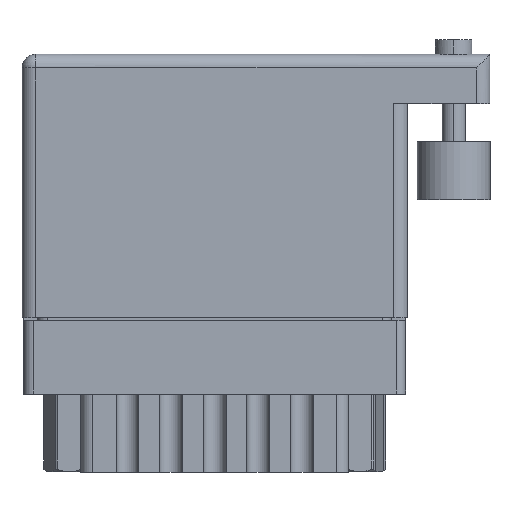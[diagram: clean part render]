
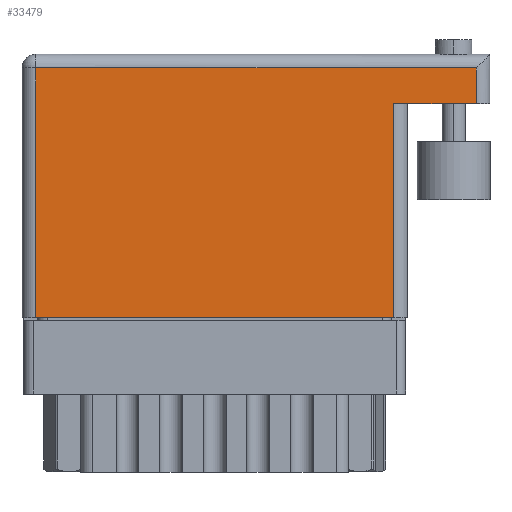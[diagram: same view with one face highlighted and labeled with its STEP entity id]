
A CAD part, front view. The second image highlights one B-rep face of the part: STEP entity #33479.
In plain terms, the highlighted face is planar.
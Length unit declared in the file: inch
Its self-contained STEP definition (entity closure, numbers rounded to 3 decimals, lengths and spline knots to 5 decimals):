
#558 = ORIENTED_EDGE ( 'NONE', *, *, #15516, .T. ) ;
#745 = CARTESIAN_POINT ( 'NONE',  ( 0.047, 0., 0. ) ) ;
#746 = VECTOR ( 'NONE', #2773, 39.37008 ) ;
#1311 = CARTESIAN_POINT ( 'NONE',  ( 1.562, 0.736, 0. ) ) ;
#1581 = FACE_OUTER_BOUND ( 'NONE', #8295, .T. ) ;
#2638 = VECTOR ( 'NONE', #4875, 39.37008 ) ;
#2724 = ORIENTED_EDGE ( 'NONE', *, *, #6875, .T. ) ;
#2773 = DIRECTION ( 'NONE',  ( -1., 0., 0. ) ) ;
#3708 = VERTEX_POINT ( 'NONE', #17145 ) ;
#3915 = LINE ( 'NONE', #11828, #11677 ) ;
#4875 = DIRECTION ( 'NONE',  ( 1., 0., 0. ) ) ;
#6190 = DIRECTION ( 'NONE',  ( 0., -1., 0. ) ) ;
#6875 = EDGE_CURVE ( 'NONE', #28937, #33581, #33011, .T. ) ;
#8295 = EDGE_LOOP ( 'NONE', ( #2724, #34405, #11783, #15850, #558, #21733 ) ) ;
#8305 = CARTESIAN_POINT ( 'NONE',  ( 1.609, 0.736, 0. ) ) ;
#9118 = CARTESIAN_POINT ( 'NONE',  ( 0., 0.859, 0. ) ) ;
#9911 = CARTESIAN_POINT ( 'NONE',  ( 0., 0.906, 0. ) ) ;
#11050 = LINE ( 'NONE', #9118, #26688 ) ;
#11677 = VECTOR ( 'NONE', #17539, 39.37008 ) ;
#11783 = ORIENTED_EDGE ( 'NONE', *, *, #16370, .F. ) ;
#11828 = CARTESIAN_POINT ( 'NONE',  ( 1.562, 0.906, 0. ) ) ;
#12876 = VERTEX_POINT ( 'NONE', #16532 ) ;
#14589 = LINE ( 'NONE', #8305, #746 ) ;
#15516 = EDGE_CURVE ( 'NONE', #3708, #27680, #11050, .T. ) ;
#15619 = DIRECTION ( 'NONE',  ( 0., 0., -1. ) ) ;
#15850 = ORIENTED_EDGE ( 'NONE', *, *, #25641, .T. ) ;
#15923 = AXIS2_PLACEMENT_3D ( 'NONE', #9911, #15619, #21220 ) ;
#16338 = LINE ( 'NONE', #27416, #28926 ) ;
#16370 = EDGE_CURVE ( 'NONE', #19627, #12876, #14589, .T. ) ;
#16532 = CARTESIAN_POINT ( 'NONE',  ( 1.278, 0.736, 0. ) ) ;
#17021 = PLANE ( 'NONE',  #15923 ) ;
#17145 = CARTESIAN_POINT ( 'NONE',  ( 1.562, 0.859, 0. ) ) ;
#17539 = DIRECTION ( 'NONE',  ( 0., 1., 0. ) ) ;
#18424 = CARTESIAN_POINT ( 'NONE',  ( 1.278, 0., 0. ) ) ;
#18737 = CARTESIAN_POINT ( 'NONE',  ( 0.047, 0., 0. ) ) ;
#19627 = VERTEX_POINT ( 'NONE', #1311 ) ;
#21220 = DIRECTION ( 'NONE',  ( -1., 0., 0. ) ) ;
#21733 = ORIENTED_EDGE ( 'NONE', *, *, #23519, .T. ) ;
#23519 = EDGE_CURVE ( 'NONE', #27680, #28937, #23958, .T. ) ;
#23958 = LINE ( 'NONE', #745, #25241 ) ;
#24532 = CARTESIAN_POINT ( 'NONE',  ( 0.047, 0.859, 0. ) ) ;
#25241 = VECTOR ( 'NONE', #6190, 39.37008 ) ;
#25641 = EDGE_CURVE ( 'NONE', #19627, #3708, #3915, .T. ) ;
#26688 = VECTOR ( 'NONE', #28174, 39.37008 ) ;
#27416 = CARTESIAN_POINT ( 'NONE',  ( 1.278, 0.736, 0. ) ) ;
#27680 = VERTEX_POINT ( 'NONE', #24532 ) ;
#27748 = EDGE_CURVE ( 'NONE', #33581, #12876, #16338, .T. ) ;
#28174 = DIRECTION ( 'NONE',  ( -1., 0., 0. ) ) ;
#28926 = VECTOR ( 'NONE', #30322, 39.37008 ) ;
#28937 = VERTEX_POINT ( 'NONE', #18737 ) ;
#30322 = DIRECTION ( 'NONE',  ( 0., 1., 0. ) ) ;
#33011 = LINE ( 'NONE', #33124, #2638 ) ;
#33124 = CARTESIAN_POINT ( 'NONE',  ( 0., 0., 0. ) ) ;
#33479 = ADVANCED_FACE ( 'NONE', ( #1581 ), #17021, .F. ) ;
#33581 = VERTEX_POINT ( 'NONE', #18424 ) ;
#34405 = ORIENTED_EDGE ( 'NONE', *, *, #27748, .T. ) ;
